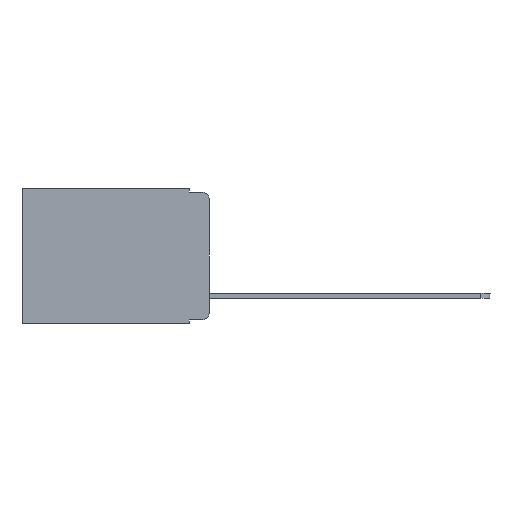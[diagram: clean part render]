
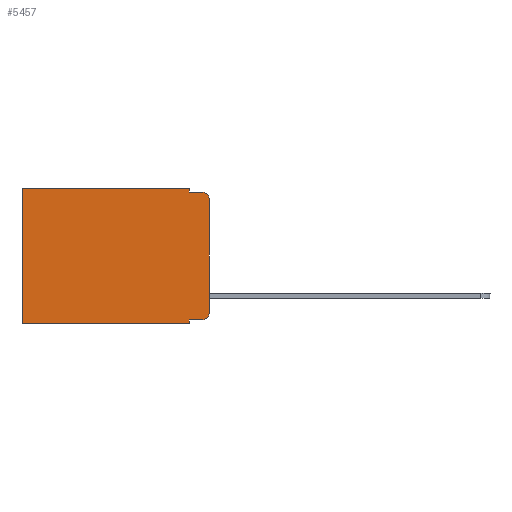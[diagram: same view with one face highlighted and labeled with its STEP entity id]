
A CAD part, left-side view. The second image highlights one B-rep face of the part: STEP entity #5457.
In plain terms, the highlighted planar face has unit normal (-1, 0, 0).
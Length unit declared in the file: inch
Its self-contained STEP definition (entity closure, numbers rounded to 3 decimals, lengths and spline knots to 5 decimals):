
#208 = EDGE_CURVE ( 'NONE', #4751, #10530, #7391, .T. ) ;
#279 = LINE ( 'NONE', #2027, #7301 ) ;
#326 = CARTESIAN_POINT ( 'NONE',  ( 0.298, 0.02, -0.333 ) ) ;
#471 = DIRECTION ( 'NONE',  ( -1., 0., 0. ) ) ;
#777 = VECTOR ( 'NONE', #7925, 39.37008 ) ;
#975 = CARTESIAN_POINT ( 'NONE',  ( 0.298, 0.051, 0. ) ) ;
#1122 = VERTEX_POINT ( 'NONE', #6431 ) ;
#1194 = VERTEX_POINT ( 'NONE', #9239 ) ;
#1335 = EDGE_CURVE ( 'NONE', #7128, #6388, #10380, .T. ) ;
#1361 = CARTESIAN_POINT ( 'NONE',  ( 0.298, 0.051, -0.333 ) ) ;
#1411 = ORIENTED_EDGE ( 'NONE', *, *, #9016, .T. ) ;
#1459 = AXIS2_PLACEMENT_3D ( 'NONE', #1587, #2457, #5940 ) ;
#1587 = CARTESIAN_POINT ( 'NONE',  ( 0.298, 0.02, -0.313 ) ) ;
#1658 = ORIENTED_EDGE ( 'NONE', *, *, #4726, .F. ) ;
#1980 = DIRECTION ( 'NONE',  ( 0., 0., -1. ) ) ;
#2027 = CARTESIAN_POINT ( 'NONE',  ( 0.298, 0.051, -0.01 ) ) ;
#2140 = DIRECTION ( 'NONE',  ( 0., -1., 0. ) ) ;
#2193 = DIRECTION ( 'NONE',  ( 0., 0., -1. ) ) ;
#2352 = ORIENTED_EDGE ( 'NONE', *, *, #11100, .F. ) ;
#2394 = DIRECTION ( 'NONE',  ( 0., 0., -1. ) ) ;
#2457 = DIRECTION ( 'NONE',  ( -1., 0., 0. ) ) ;
#2476 = EDGE_CURVE ( 'NONE', #1194, #7128, #5834, .T. ) ;
#2641 = EDGE_CURVE ( 'NONE', #9535, #10530, #5093, .T. ) ;
#2861 = CIRCLE ( 'NONE', #8635, 0.02 ) ;
#2987 = ORIENTED_EDGE ( 'NONE', *, *, #2641, .F. ) ;
#3070 = CARTESIAN_POINT ( 'NONE',  ( 0.298, 0., 0. ) ) ;
#3692 = VERTEX_POINT ( 'NONE', #10810 ) ;
#4027 = CARTESIAN_POINT ( 'NONE',  ( 0.298, 0.051, -0.01 ) ) ;
#4090 = CARTESIAN_POINT ( 'NONE',  ( 0.298, 0., 0. ) ) ;
#4205 = LINE ( 'NONE', #4090, #9540 ) ;
#4261 = VERTEX_POINT ( 'NONE', #7601 ) ;
#4299 = CARTESIAN_POINT ( 'NONE',  ( 0.298, 0.473, 0. ) ) ;
#4312 = CARTESIAN_POINT ( 'NONE',  ( 0.298, 0., -0.343 ) ) ;
#4531 = DIRECTION ( 'NONE',  ( 0., 0., -1. ) ) ;
#4706 = CARTESIAN_POINT ( 'NONE',  ( 0.298, 0.051, 0. ) ) ;
#4726 = EDGE_CURVE ( 'NONE', #4261, #6388, #10592, .T. ) ;
#4751 = VERTEX_POINT ( 'NONE', #4299 ) ;
#5093 = LINE ( 'NONE', #4312, #777 ) ;
#5226 = EDGE_LOOP ( 'NONE', ( #1658, #1411, #10732, #2352, #8203, #10453, #2987, #7300, #7918, #6436 ) ) ;
#5457 = ADVANCED_FACE ( 'NONE', ( #10214 ), #5683, .F. ) ;
#5500 = EDGE_CURVE ( 'NONE', #9000, #3692, #279, .T. ) ;
#5569 = DIRECTION ( 'NONE',  ( 1., 0., 0. ) ) ;
#5655 = VECTOR ( 'NONE', #4531, 39.37008 ) ;
#5680 = LINE ( 'NONE', #4706, #5687 ) ;
#5683 = PLANE ( 'NONE',  #8604 ) ;
#5687 = VECTOR ( 'NONE', #10868, 39.37008 ) ;
#5834 = LINE ( 'NONE', #1361, #9332 ) ;
#5940 = DIRECTION ( 'NONE',  ( 0., 0., -1. ) ) ;
#6119 = VECTOR ( 'NONE', #1980, 39.37008 ) ;
#6388 = VERTEX_POINT ( 'NONE', #10119 ) ;
#6431 = CARTESIAN_POINT ( 'NONE',  ( 0.298, 0.051, 0. ) ) ;
#6436 = ORIENTED_EDGE ( 'NONE', *, *, #1335, .T. ) ;
#6771 = DIRECTION ( 'NONE',  ( 0., 1., 0. ) ) ;
#6929 = CARTESIAN_POINT ( 'NONE',  ( 0.298, 0., 0. ) ) ;
#7128 = VERTEX_POINT ( 'NONE', #326 ) ;
#7300 = ORIENTED_EDGE ( 'NONE', *, *, #9226, .F. ) ;
#7301 = VECTOR ( 'NONE', #2140, 39.37008 ) ;
#7391 = LINE ( 'NONE', #10821, #6119 ) ;
#7601 = CARTESIAN_POINT ( 'NONE',  ( 0.298, 0., -0.03 ) ) ;
#7762 = EDGE_CURVE ( 'NONE', #1122, #4751, #4205, .T. ) ;
#7918 = ORIENTED_EDGE ( 'NONE', *, *, #2476, .T. ) ;
#7925 = DIRECTION ( 'NONE',  ( 0., 1., 0. ) ) ;
#7966 = CARTESIAN_POINT ( 'NONE',  ( 0.298, 0.473, -0.343 ) ) ;
#8203 = ORIENTED_EDGE ( 'NONE', *, *, #7762, .T. ) ;
#8447 = CARTESIAN_POINT ( 'NONE',  ( 0.298, 0.02, -0.03 ) ) ;
#8604 = AXIS2_PLACEMENT_3D ( 'NONE', #3070, #5569, #2193 ) ;
#8635 = AXIS2_PLACEMENT_3D ( 'NONE', #8447, #471, #10009 ) ;
#8955 = LINE ( 'NONE', #975, #5655 ) ;
#9000 = VERTEX_POINT ( 'NONE', #4027 ) ;
#9016 = EDGE_CURVE ( 'NONE', #4261, #3692, #2861, .T. ) ;
#9226 = EDGE_CURVE ( 'NONE', #1194, #9535, #8955, .T. ) ;
#9239 = CARTESIAN_POINT ( 'NONE',  ( 0.298, 0.051, -0.333 ) ) ;
#9332 = VECTOR ( 'NONE', #11019, 39.37008 ) ;
#9535 = VERTEX_POINT ( 'NONE', #11268 ) ;
#9540 = VECTOR ( 'NONE', #6771, 39.37008 ) ;
#10009 = DIRECTION ( 'NONE',  ( 0., 0., -1. ) ) ;
#10119 = CARTESIAN_POINT ( 'NONE',  ( 0.298, 0., -0.313 ) ) ;
#10214 = FACE_OUTER_BOUND ( 'NONE', #5226, .T. ) ;
#10380 = CIRCLE ( 'NONE', #1459, 0.02 ) ;
#10441 = VECTOR ( 'NONE', #2394, 39.37008 ) ;
#10453 = ORIENTED_EDGE ( 'NONE', *, *, #208, .T. ) ;
#10530 = VERTEX_POINT ( 'NONE', #7966 ) ;
#10592 = LINE ( 'NONE', #6929, #10441 ) ;
#10732 = ORIENTED_EDGE ( 'NONE', *, *, #5500, .F. ) ;
#10810 = CARTESIAN_POINT ( 'NONE',  ( 0.298, 0.02, -0.01 ) ) ;
#10821 = CARTESIAN_POINT ( 'NONE',  ( 0.298, 0.473, 0. ) ) ;
#10868 = DIRECTION ( 'NONE',  ( 0., 0., -1. ) ) ;
#11019 = DIRECTION ( 'NONE',  ( 0., -1., 0. ) ) ;
#11100 = EDGE_CURVE ( 'NONE', #1122, #9000, #5680, .T. ) ;
#11268 = CARTESIAN_POINT ( 'NONE',  ( 0.298, 0.051, -0.343 ) ) ;
